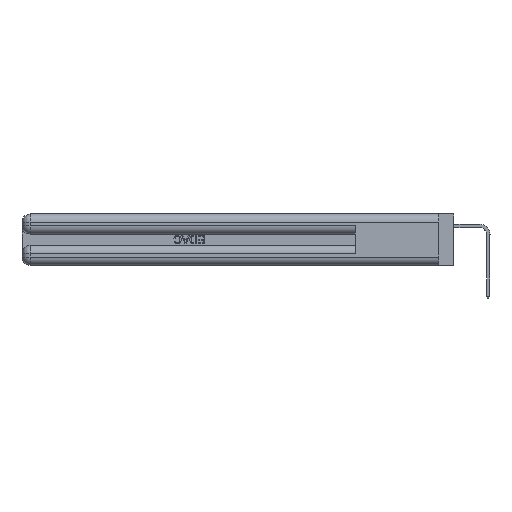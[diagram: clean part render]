
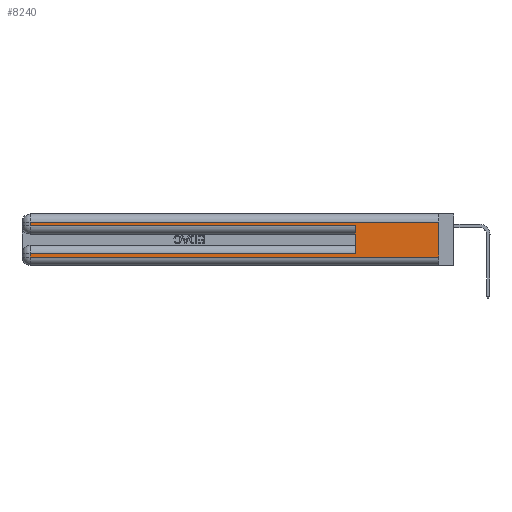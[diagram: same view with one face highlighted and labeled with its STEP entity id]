
A CAD part, left-side view. The second image highlights one B-rep face of the part: STEP entity #8240.
In plain terms, the highlighted planar face has unit normal (-1, 0, 0).
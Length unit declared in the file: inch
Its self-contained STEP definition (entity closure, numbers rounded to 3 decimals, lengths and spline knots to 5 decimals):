
#828 = EDGE_CURVE ( 'NONE', #40198, #21158, #30549, .T. ) ;
#1349 = DIRECTION ( 'NONE',  ( 0., 0., -1. ) ) ;
#1350 = CARTESIAN_POINT ( 'NONE',  ( 0., 0., 0.085 ) ) ;
#1386 = DIRECTION ( 'NONE',  ( 0., -1., 0. ) ) ;
#1848 = CARTESIAN_POINT ( 'NONE',  ( 0., 0.6, 0.145 ) ) ;
#2957 = LINE ( 'NONE', #7166, #30653 ) ;
#3597 = LINE ( 'NONE', #1848, #42688 ) ;
#3817 = ORIENTED_EDGE ( 'NONE', *, *, #13666, .T. ) ;
#3913 = VECTOR ( 'NONE', #1349, 39.37008 ) ;
#4234 = CARTESIAN_POINT ( 'NONE',  ( 0., 0.6, 0.085 ) ) ;
#5416 = ORIENTED_EDGE ( 'NONE', *, *, #10757, .F. ) ;
#6496 = VECTOR ( 'NONE', #22137, 39.37008 ) ;
#7166 = CARTESIAN_POINT ( 'NONE',  ( 0., 0., 0.06 ) ) ;
#8240 = ADVANCED_FACE ( 'NONE', ( #29954 ), #36500, .F. ) ;
#8731 = EDGE_CURVE ( 'NONE', #33976, #30147, #36618, .T. ) ;
#9637 = VERTEX_POINT ( 'NONE', #21779 ) ;
#10757 = EDGE_CURVE ( 'NONE', #23048, #39693, #3597, .T. ) ;
#13214 = DIRECTION ( 'NONE',  ( 0., 0., -1. ) ) ;
#13361 = ORIENTED_EDGE ( 'NONE', *, *, #27485, .T. ) ;
#13666 = EDGE_CURVE ( 'NONE', #40198, #33976, #15453, .T. ) ;
#15453 = LINE ( 'NONE', #28679, #6496 ) ;
#15954 = ORIENTED_EDGE ( 'NONE', *, *, #28832, .T. ) ;
#17297 = DIRECTION ( 'NONE',  ( 0., -1., 0. ) ) ;
#17490 = VECTOR ( 'NONE', #1386, 39.37008 ) ;
#19811 = CARTESIAN_POINT ( 'NONE',  ( 0., 2.94, 0.37 ) ) ;
#20016 = DIRECTION ( 'NONE',  ( 0., 0., -1. ) ) ;
#20108 = CARTESIAN_POINT ( 'NONE',  ( 0., 2.94, 0.37 ) ) ;
#20129 = VECTOR ( 'NONE', #26800, 39.37008 ) ;
#20599 = ORIENTED_EDGE ( 'NONE', *, *, #23752, .T. ) ;
#21158 = VERTEX_POINT ( 'NONE', #22347 ) ;
#21779 = CARTESIAN_POINT ( 'NONE',  ( 0., 2.94, 0.06 ) ) ;
#22040 = CARTESIAN_POINT ( 'NONE',  ( 0., 2.94, 0.285 ) ) ;
#22137 = DIRECTION ( 'NONE',  ( 0., 1., 0. ) ) ;
#22347 = CARTESIAN_POINT ( 'NONE',  ( 0., 0., 0.06 ) ) ;
#23048 = VERTEX_POINT ( 'NONE', #4234 ) ;
#23425 = CARTESIAN_POINT ( 'NONE',  ( 0., 2.94, 0.085 ) ) ;
#23752 = EDGE_CURVE ( 'NONE', #30147, #39693, #26338, .T. ) ;
#24753 = DIRECTION ( 'NONE',  ( 0., 1., 0. ) ) ;
#24794 = CARTESIAN_POINT ( 'NONE',  ( 0., 0., 0.285 ) ) ;
#25256 = DIRECTION ( 'NONE',  ( 0., 0., 1. ) ) ;
#26222 = AXIS2_PLACEMENT_3D ( 'NONE', #43064, #39835, #20016 ) ;
#26338 = LINE ( 'NONE', #24794, #17490 ) ;
#26800 = DIRECTION ( 'NONE',  ( 0., 0., -1. ) ) ;
#26983 = LINE ( 'NONE', #1350, #36790 ) ;
#27485 = EDGE_CURVE ( 'NONE', #9637, #21158, #2957, .T. ) ;
#28679 = CARTESIAN_POINT ( 'NONE',  ( 0., 0., 0.31 ) ) ;
#28832 = EDGE_CURVE ( 'NONE', #23048, #30432, #26983, .T. ) ;
#28906 = EDGE_LOOP ( 'NONE', ( #36617, #3817, #35608, #20599, #5416, #15954, #36214, #13361 ) ) ;
#29954 = FACE_OUTER_BOUND ( 'NONE', #28906, .T. ) ;
#30147 = VERTEX_POINT ( 'NONE', #22040 ) ;
#30432 = VERTEX_POINT ( 'NONE', #23425 ) ;
#30549 = LINE ( 'NONE', #31267, #3913 ) ;
#30653 = VECTOR ( 'NONE', #17297, 39.37008 ) ;
#31267 = CARTESIAN_POINT ( 'NONE',  ( 0., 0., 0.37 ) ) ;
#33976 = VERTEX_POINT ( 'NONE', #35445 ) ;
#34751 = CARTESIAN_POINT ( 'NONE',  ( 0., 0.6, 0.285 ) ) ;
#35445 = CARTESIAN_POINT ( 'NONE',  ( 0., 2.94, 0.31 ) ) ;
#35598 = VECTOR ( 'NONE', #13214, 39.37008 ) ;
#35608 = ORIENTED_EDGE ( 'NONE', *, *, #8731, .T. ) ;
#36214 = ORIENTED_EDGE ( 'NONE', *, *, #36439, .T. ) ;
#36439 = EDGE_CURVE ( 'NONE', #30432, #9637, #37736, .T. ) ;
#36500 = PLANE ( 'NONE',  #26222 ) ;
#36617 = ORIENTED_EDGE ( 'NONE', *, *, #828, .F. ) ;
#36618 = LINE ( 'NONE', #19811, #35598 ) ;
#36790 = VECTOR ( 'NONE', #24753, 39.37008 ) ;
#37736 = LINE ( 'NONE', #20108, #20129 ) ;
#39693 = VERTEX_POINT ( 'NONE', #34751 ) ;
#39835 = DIRECTION ( 'NONE',  ( 1., 0., 0. ) ) ;
#40198 = VERTEX_POINT ( 'NONE', #40488 ) ;
#40488 = CARTESIAN_POINT ( 'NONE',  ( 0., 0., 0.31 ) ) ;
#42688 = VECTOR ( 'NONE', #25256, 39.37008 ) ;
#43064 = CARTESIAN_POINT ( 'NONE',  ( 0., 0., 0.37 ) ) ;
